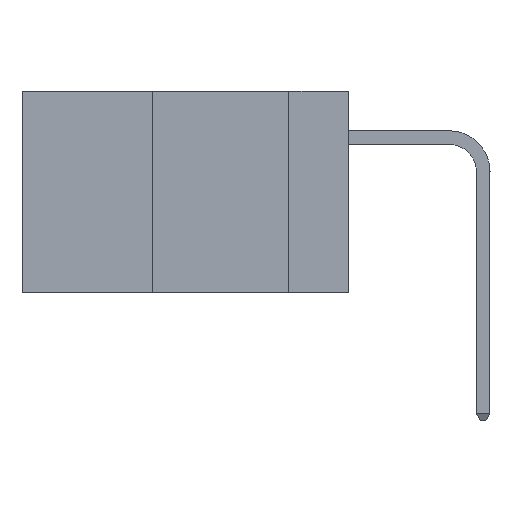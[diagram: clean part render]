
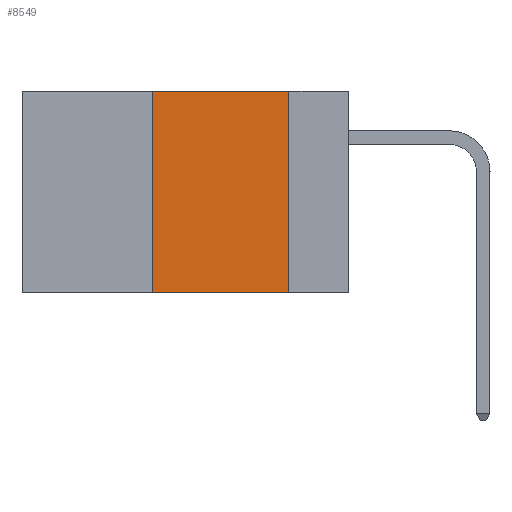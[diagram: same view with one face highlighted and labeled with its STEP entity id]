
A CAD part, left-side view. The second image highlights one B-rep face of the part: STEP entity #8549.
In plain terms, the highlighted planar face has unit normal (-1, 0, 0).
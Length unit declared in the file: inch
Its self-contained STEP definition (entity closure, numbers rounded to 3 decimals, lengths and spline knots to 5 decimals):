
#380 = CARTESIAN_POINT ( 'NONE',  ( 0., 0.6, -0.37 ) ) ;
#1208 = VERTEX_POINT ( 'NONE', #38589 ) ;
#3534 = ORIENTED_EDGE ( 'NONE', *, *, #41455, .F. ) ;
#4018 = CARTESIAN_POINT ( 'NONE',  ( 0., 0.36, 0. ) ) ;
#5595 = ORIENTED_EDGE ( 'NONE', *, *, #7113, .F. ) ;
#7113 = EDGE_CURVE ( 'NONE', #41510, #44542, #30026, .T. ) ;
#7584 = CARTESIAN_POINT ( 'NONE',  ( 0., 0.11, 0. ) ) ;
#7638 = DIRECTION ( 'NONE',  ( 0., 0., -1. ) ) ;
#8190 = VECTOR ( 'NONE', #44100, 39.37008 ) ;
#8515 = FACE_OUTER_BOUND ( 'NONE', #30078, .T. ) ;
#8549 = ADVANCED_FACE ( 'NONE', ( #8515 ), #11003, .F. ) ;
#10030 = CARTESIAN_POINT ( 'NONE',  ( 0., 0.6, 0. ) ) ;
#11003 = PLANE ( 'NONE',  #28436 ) ;
#12480 = LINE ( 'NONE', #39720, #35826 ) ;
#13652 = VERTEX_POINT ( 'NONE', #19016 ) ;
#13759 = DIRECTION ( 'NONE',  ( 0., 0., 1. ) ) ;
#15523 = CARTESIAN_POINT ( 'NONE',  ( 0., 0.11, 0. ) ) ;
#15821 = LINE ( 'NONE', #380, #34672 ) ;
#17843 = EDGE_CURVE ( 'NONE', #13652, #41510, #12480, .T. ) ;
#19016 = CARTESIAN_POINT ( 'NONE',  ( 0., 0.36, -0.37 ) ) ;
#21335 = LINE ( 'NONE', #15523, #8190 ) ;
#25678 = CARTESIAN_POINT ( 'NONE',  ( 0., 0.6, 0. ) ) ;
#27064 = DIRECTION ( 'NONE',  ( 0., -1., 0. ) ) ;
#27789 = ORIENTED_EDGE ( 'NONE', *, *, #38879, .T. ) ;
#27927 = DIRECTION ( 'NONE',  ( 0., -1., 0. ) ) ;
#28436 = AXIS2_PLACEMENT_3D ( 'NONE', #25678, #40624, #7638 ) ;
#30026 = LINE ( 'NONE', #10030, #42575 ) ;
#30078 = EDGE_LOOP ( 'NONE', ( #3534, #5595, #36024, #27789 ) ) ;
#34672 = VECTOR ( 'NONE', #27064, 39.37008 ) ;
#35826 = VECTOR ( 'NONE', #13759, 39.37008 ) ;
#36024 = ORIENTED_EDGE ( 'NONE', *, *, #17843, .F. ) ;
#38589 = CARTESIAN_POINT ( 'NONE',  ( 0., 0.11, -0.37 ) ) ;
#38879 = EDGE_CURVE ( 'NONE', #13652, #1208, #15821, .T. ) ;
#39720 = CARTESIAN_POINT ( 'NONE',  ( 0., 0.36, 0. ) ) ;
#40624 = DIRECTION ( 'NONE',  ( 1., 0., 0. ) ) ;
#41455 = EDGE_CURVE ( 'NONE', #44542, #1208, #21335, .T. ) ;
#41510 = VERTEX_POINT ( 'NONE', #4018 ) ;
#42575 = VECTOR ( 'NONE', #27927, 39.37008 ) ;
#44100 = DIRECTION ( 'NONE',  ( 0., 0., -1. ) ) ;
#44542 = VERTEX_POINT ( 'NONE', #7584 ) ;
